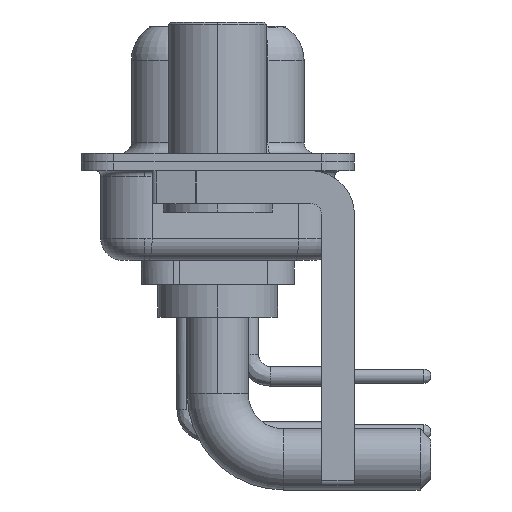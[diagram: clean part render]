
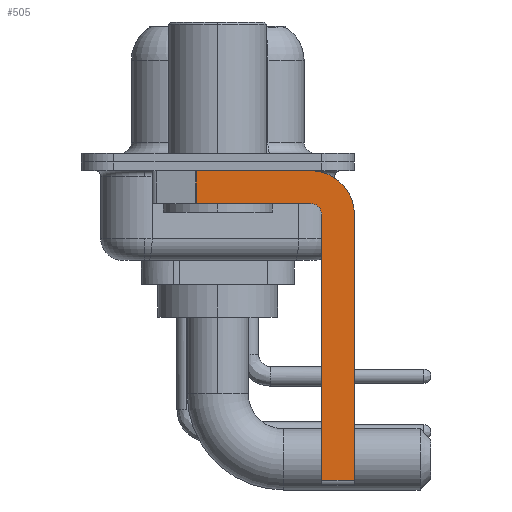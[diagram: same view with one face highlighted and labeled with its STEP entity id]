
A CAD part, left-side view. The second image highlights one B-rep face of the part: STEP entity #505.
In plain terms, the highlighted planar face has unit normal (-1, 0, 0).
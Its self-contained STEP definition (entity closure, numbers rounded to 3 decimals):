
#31 = EDGE_CURVE ( 'NONE', #16872, #3697, #3321, .T. ) ;
#505 = ADVANCED_FACE ( 'NONE', ( #21620 ), #14834, .F. ) ;
#737 = EDGE_CURVE ( 'NONE', #4683, #12420, #19182, .T. ) ;
#946 = CARTESIAN_POINT ( 'NONE',  ( -2.9, 0.978, -1.9 ) ) ;
#1535 = VERTEX_POINT ( 'NONE', #946 ) ;
#1823 = VERTEX_POINT ( 'NONE', #10936 ) ;
#3145 = ORIENTED_EDGE ( 'NONE', *, *, #8157, .F. ) ;
#3276 = EDGE_CURVE ( 'NONE', #4223, #1535, #5879, .T. ) ;
#3321 = CIRCLE ( 'NONE', #7723, 0.5 ) ;
#3697 = VERTEX_POINT ( 'NONE', #13684 ) ;
#4214 = DIRECTION ( 'NONE',  ( 0., 1., 0. ) ) ;
#4223 = VERTEX_POINT ( 'NONE', #14322 ) ;
#4323 = CARTESIAN_POINT ( 'NONE',  ( -2.9, -4.25, -1.9 ) ) ;
#4375 = CARTESIAN_POINT ( 'NONE',  ( -2.9, -4.25, -2.4 ) ) ;
#4473 = VECTOR ( 'NONE', #19662, 1000. ) ;
#4683 = VERTEX_POINT ( 'NONE', #22378 ) ;
#4825 = CARTESIAN_POINT ( 'NONE',  ( -2.9, -6.25, -2.4 ) ) ;
#4853 = EDGE_CURVE ( 'NONE', #3697, #1535, #8006, .T. ) ;
#5335 = ORIENTED_EDGE ( 'NONE', *, *, #13730, .T. ) ;
#5555 = DIRECTION ( 'NONE',  ( 0., 0., 1. ) ) ;
#5879 = LINE ( 'NONE', #10943, #20633 ) ;
#6539 = ORIENTED_EDGE ( 'NONE', *, *, #4853, .F. ) ;
#7516 = CARTESIAN_POINT ( 'NONE',  ( -2.9, -4.25, -2.4 ) ) ;
#7542 = ORIENTED_EDGE ( 'NONE', *, *, #737, .F. ) ;
#7723 = AXIS2_PLACEMENT_3D ( 'NONE', #7516, #21309, #5555 ) ;
#8006 = LINE ( 'NONE', #4323, #19973 ) ;
#8157 = EDGE_CURVE ( 'NONE', #9519, #4683, #14226, .T. ) ;
#8939 = CARTESIAN_POINT ( 'NONE',  ( -2.9, -4.75, -2.4 ) ) ;
#9405 = CARTESIAN_POINT ( 'NONE',  ( -2.9, -4.75, -14.8 ) ) ;
#9519 = VERTEX_POINT ( 'NONE', #13570 ) ;
#9637 = DIRECTION ( 'NONE',  ( 0., 0., -1. ) ) ;
#9858 = LINE ( 'NONE', #9405, #14910 ) ;
#10013 = ORIENTED_EDGE ( 'NONE', *, *, #14195, .F. ) ;
#10618 = AXIS2_PLACEMENT_3D ( 'NONE', #4375, #13010, #12892 ) ;
#10936 = CARTESIAN_POINT ( 'NONE',  ( -2.9, -4.75, -14.55 ) ) ;
#10943 = CARTESIAN_POINT ( 'NONE',  ( -2.9, 0.978, -1.9 ) ) ;
#10999 = ORIENTED_EDGE ( 'NONE', *, *, #3276, .T. ) ;
#11063 = EDGE_CURVE ( 'NONE', #1823, #16872, #9858, .T. ) ;
#11401 = ORIENTED_EDGE ( 'NONE', *, *, #31, .F. ) ;
#11713 = CARTESIAN_POINT ( 'NONE',  ( -2.9, -4.25, -2.4 ) ) ;
#11755 = VECTOR ( 'NONE', #20469, 1000. ) ;
#12304 = DIRECTION ( 'NONE',  ( 0., -1., 0. ) ) ;
#12420 = VERTEX_POINT ( 'NONE', #19088 ) ;
#12892 = DIRECTION ( 'NONE',  ( 0., 0., -1. ) ) ;
#12896 = EDGE_LOOP ( 'NONE', ( #10013, #10999, #6539, #11401, #21475, #5335, #7542, #3145 ) ) ;
#13010 = DIRECTION ( 'NONE',  ( 1., 0., 0. ) ) ;
#13570 = CARTESIAN_POINT ( 'NONE',  ( -2.9, -4.25, -0.4 ) ) ;
#13684 = CARTESIAN_POINT ( 'NONE',  ( -2.9, -4.25, -1.9 ) ) ;
#13730 = EDGE_CURVE ( 'NONE', #1823, #12420, #15976, .T. ) ;
#14195 = EDGE_CURVE ( 'NONE', #4223, #9519, #14335, .T. ) ;
#14226 = CIRCLE ( 'NONE', #17884, 2. ) ;
#14322 = CARTESIAN_POINT ( 'NONE',  ( -2.9, 0.978, -0.4 ) ) ;
#14335 = LINE ( 'NONE', #20910, #22472 ) ;
#14834 = PLANE ( 'NONE',  #10618 ) ;
#14910 = VECTOR ( 'NONE', #18463, 1000. ) ;
#15976 = LINE ( 'NONE', #16085, #4473 ) ;
#16085 = CARTESIAN_POINT ( 'NONE',  ( -2.9, -4.25, -14.55 ) ) ;
#16872 = VERTEX_POINT ( 'NONE', #8939 ) ;
#17834 = DIRECTION ( 'NONE',  ( 0., 0., -1. ) ) ;
#17884 = AXIS2_PLACEMENT_3D ( 'NONE', #11713, #18362, #9637 ) ;
#18362 = DIRECTION ( 'NONE',  ( 1., 0., 0. ) ) ;
#18463 = DIRECTION ( 'NONE',  ( 0., 0., 1. ) ) ;
#19088 = CARTESIAN_POINT ( 'NONE',  ( -2.9, -6.25, -14.55 ) ) ;
#19182 = LINE ( 'NONE', #4825, #11755 ) ;
#19662 = DIRECTION ( 'NONE',  ( 0., -1., 0. ) ) ;
#19973 = VECTOR ( 'NONE', #4214, 1000. ) ;
#20469 = DIRECTION ( 'NONE',  ( 0., 0., -1. ) ) ;
#20633 = VECTOR ( 'NONE', #17834, 1000. ) ;
#20910 = CARTESIAN_POINT ( 'NONE',  ( -2.9, 3., -0.4 ) ) ;
#21309 = DIRECTION ( 'NONE',  ( -1., 0., 0. ) ) ;
#21475 = ORIENTED_EDGE ( 'NONE', *, *, #11063, .F. ) ;
#21620 = FACE_OUTER_BOUND ( 'NONE', #12896, .T. ) ;
#22378 = CARTESIAN_POINT ( 'NONE',  ( -2.9, -6.25, -2.4 ) ) ;
#22472 = VECTOR ( 'NONE', #12304, 1000. ) ;
